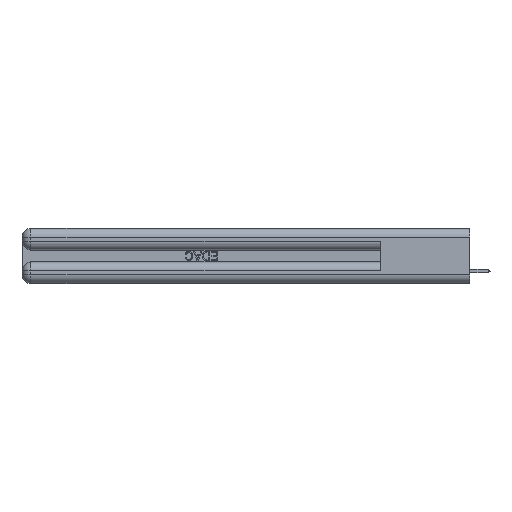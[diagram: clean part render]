
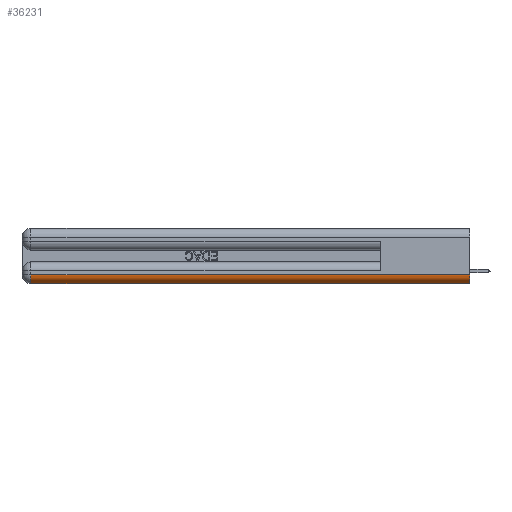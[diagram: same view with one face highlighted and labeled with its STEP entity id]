
A CAD part, left-side view. The second image highlights one B-rep face of the part: STEP entity #36231.
In plain terms, the highlighted cylindrical face has radius 1.524 mm (diameter 3.048 mm), a partial arc.
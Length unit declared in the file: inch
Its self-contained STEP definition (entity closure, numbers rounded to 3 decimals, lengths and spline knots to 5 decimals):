
#555 = ORIENTED_EDGE ( 'NONE', *, *, #50230, .F. ) ;
#2006 = ORIENTED_EDGE ( 'NONE', *, *, #2373, .F. ) ;
#2373 = EDGE_CURVE ( 'NONE', #53532, #31909, #33395, .T. ) ;
#4816 = FACE_OUTER_BOUND ( 'NONE', #53040, .T. ) ;
#6540 = AXIS2_PLACEMENT_3D ( 'NONE', #38392, #30571, #35297 ) ;
#10177 = LINE ( 'NONE', #23561, #53382 ) ;
#12842 = EDGE_CURVE ( 'NONE', #32755, #31556, #35725, .T. ) ;
#13380 = CARTESIAN_POINT ( 'NONE',  ( 0., 2.94, 0.06 ) ) ;
#17430 = AXIS2_PLACEMENT_3D ( 'NONE', #41759, #21286, #29860 ) ;
#18012 = ORIENTED_EDGE ( 'NONE', *, *, #12842, .F. ) ;
#18127 = CARTESIAN_POINT ( 'NONE',  ( 0.06, 0., 0.06 ) ) ;
#18188 = DIRECTION ( 'NONE',  ( 0., -1., 0. ) ) ;
#21286 = DIRECTION ( 'NONE',  ( 0., 1., 0. ) ) ;
#22043 = EDGE_CURVE ( 'NONE', #31909, #32755, #43360, .T. ) ;
#23561 = CARTESIAN_POINT ( 'NONE',  ( 0.06, 3., 0. ) ) ;
#27464 = DIRECTION ( 'NONE',  ( 0., -1., 0. ) ) ;
#29854 = CARTESIAN_POINT ( 'NONE',  ( 0.06, 2.94, 0. ) ) ;
#29860 = DIRECTION ( 'NONE',  ( 0., 0., 1. ) ) ;
#30571 = DIRECTION ( 'NONE',  ( 0., 1., 0. ) ) ;
#31556 = VERTEX_POINT ( 'NONE', #45086 ) ;
#31909 = VERTEX_POINT ( 'NONE', #13380 ) ;
#32755 = VERTEX_POINT ( 'NONE', #38711 ) ;
#33395 = CIRCLE ( 'NONE', #17430, 0.06 ) ;
#35297 = DIRECTION ( 'NONE',  ( 0., 0., 1. ) ) ;
#35362 = DIRECTION ( 'NONE',  ( 0., 0., 1. ) ) ;
#35725 = CIRCLE ( 'NONE', #50620, 0.06 ) ;
#36231 = ADVANCED_FACE ( 'NONE', ( #4816 ), #36935, .T. ) ;
#36935 = CYLINDRICAL_SURFACE ( 'NONE', #6540, 0.06 ) ;
#38392 = CARTESIAN_POINT ( 'NONE',  ( 0.06, 0., 0.06 ) ) ;
#38660 = ORIENTED_EDGE ( 'NONE', *, *, #22043, .F. ) ;
#38711 = CARTESIAN_POINT ( 'NONE',  ( 0., 0., 0.06 ) ) ;
#41759 = CARTESIAN_POINT ( 'NONE',  ( 0.06, 2.94, 0.06 ) ) ;
#43360 = LINE ( 'NONE', #47562, #46031 ) ;
#45086 = CARTESIAN_POINT ( 'NONE',  ( 0.06, 0., 0. ) ) ;
#46031 = VECTOR ( 'NONE', #18188, 39.37008 ) ;
#47562 = CARTESIAN_POINT ( 'NONE',  ( 0., 0., 0.06 ) ) ;
#50230 = EDGE_CURVE ( 'NONE', #31556, #53532, #10177, .T. ) ;
#50620 = AXIS2_PLACEMENT_3D ( 'NONE', #18127, #27464, #35362 ) ;
#52293 = DIRECTION ( 'NONE',  ( 0., 1., 0. ) ) ;
#53040 = EDGE_LOOP ( 'NONE', ( #18012, #38660, #2006, #555 ) ) ;
#53382 = VECTOR ( 'NONE', #52293, 39.37008 ) ;
#53532 = VERTEX_POINT ( 'NONE', #29854 ) ;
